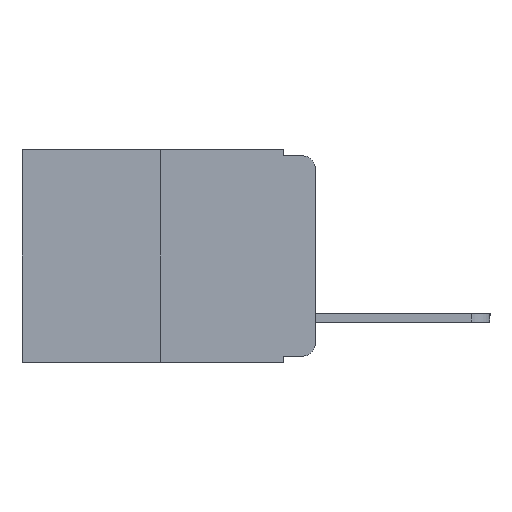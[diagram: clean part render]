
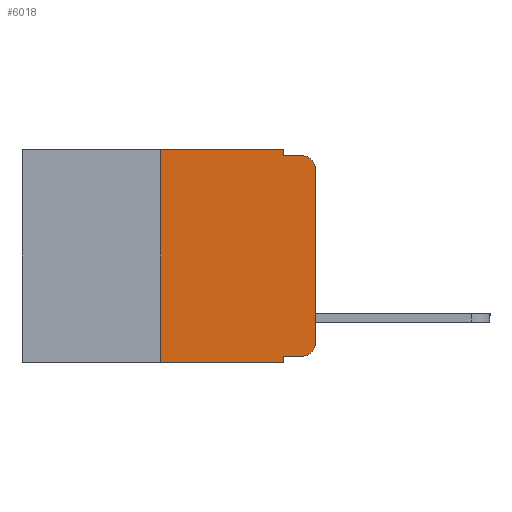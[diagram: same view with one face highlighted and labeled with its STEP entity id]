
A CAD part, left-side view. The second image highlights one B-rep face of the part: STEP entity #6018.
In plain terms, the highlighted planar face has unit normal (-1, 0, 0).
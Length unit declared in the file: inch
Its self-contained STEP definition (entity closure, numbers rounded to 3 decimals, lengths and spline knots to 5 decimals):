
#247 = ORIENTED_EDGE ( 'NONE', *, *, #2678, .F. ) ;
#1972 = LINE ( 'NONE', #10552, #6035 ) ;
#2159 = EDGE_CURVE ( 'NONE', #5291, #13339, #17502, .T. ) ;
#2194 = EDGE_CURVE ( 'NONE', #17381, #5291, #2397, .T. ) ;
#2248 = EDGE_CURVE ( 'NONE', #17381, #13971, #9463, .T. ) ;
#2251 = EDGE_CURVE ( 'NONE', #16331, #6936, #5958, .T. ) ;
#2273 = EDGE_CURVE ( 'NONE', #5850, #3228, #5027, .T. ) ;
#2397 = LINE ( 'NONE', #7109, #9899 ) ;
#2626 = CARTESIAN_POINT ( 'NONE',  ( 0., 0.473, 0. ) ) ;
#2678 = EDGE_CURVE ( 'NONE', #3228, #6550, #5731, .T. ) ;
#2682 = EDGE_CURVE ( 'NONE', #3703, #6550, #12694, .T. ) ;
#2685 = EDGE_CURVE ( 'NONE', #13339, #3703, #5261, .T. ) ;
#3228 = VERTEX_POINT ( 'NONE', #13701 ) ;
#3464 = CARTESIAN_POINT ( 'NONE',  ( 0., 0.02, -0.333 ) ) ;
#3703 = VERTEX_POINT ( 'NONE', #9690 ) ;
#3707 = CARTESIAN_POINT ( 'NONE',  ( 0., 0.051, -0.343 ) ) ;
#3826 = DIRECTION ( 'NONE',  ( 0., 0., -1. ) ) ;
#4146 = DIRECTION ( 'NONE',  ( 0., -1., 0. ) ) ;
#4925 = DIRECTION ( 'NONE',  ( 0., 0., 1. ) ) ;
#5027 = LINE ( 'NONE', #6046, #15476 ) ;
#5111 = CARTESIAN_POINT ( 'NONE',  ( 0., 0.25, 0. ) ) ;
#5170 = DIRECTION ( 'NONE',  ( 0., 0., -1. ) ) ;
#5261 = LINE ( 'NONE', #17087, #15670 ) ;
#5291 = VERTEX_POINT ( 'NONE', #3464 ) ;
#5731 = LINE ( 'NONE', #8336, #9234 ) ;
#5735 = CARTESIAN_POINT ( 'NONE',  ( 0., 0.25, 0. ) ) ;
#5850 = VERTEX_POINT ( 'NONE', #5943 ) ;
#5943 = CARTESIAN_POINT ( 'NONE',  ( 0., 0.051, 0. ) ) ;
#5949 = CARTESIAN_POINT ( 'NONE',  ( 0., 0.25, -0.343 ) ) ;
#5958 = LINE ( 'NONE', #5111, #9007 ) ;
#6018 = ADVANCED_FACE ( 'NONE', ( #11498 ), #15087, .F. ) ;
#6035 = VECTOR ( 'NONE', #9173, 39.37008 ) ;
#6046 = CARTESIAN_POINT ( 'NONE',  ( 0., 0.051, 0. ) ) ;
#6058 = CARTESIAN_POINT ( 'NONE',  ( 0., 0.051, 0. ) ) ;
#6550 = VERTEX_POINT ( 'NONE', #13350 ) ;
#6936 = VERTEX_POINT ( 'NONE', #5735 ) ;
#7101 = EDGE_CURVE ( 'NONE', #16331, #13971, #1972, .T. ) ;
#7109 = CARTESIAN_POINT ( 'NONE',  ( 0., 0.051, -0.333 ) ) ;
#7157 = VECTOR ( 'NONE', #13172, 39.37008 ) ;
#7389 = DIRECTION ( 'NONE',  ( 0., -1., 0. ) ) ;
#7745 = EDGE_LOOP ( 'NONE', ( #14069, #11121, #247, #14455, #15666, #8746, #9229, #9391, #16634, #12688 ) ) ;
#7762 = DIRECTION ( 'NONE',  ( 0., 0., -1. ) ) ;
#7802 = DIRECTION ( 'NONE',  ( -1., 0., 0. ) ) ;
#7881 = CARTESIAN_POINT ( 'NONE',  ( 0., 0.02, -0.313 ) ) ;
#8336 = CARTESIAN_POINT ( 'NONE',  ( 0., 0.051, -0.01 ) ) ;
#8705 = AXIS2_PLACEMENT_3D ( 'NONE', #2626, #15027, #15004 ) ;
#8746 = ORIENTED_EDGE ( 'NONE', *, *, #2251, .F. ) ;
#9007 = VECTOR ( 'NONE', #4925, 39.37008 ) ;
#9173 = DIRECTION ( 'NONE',  ( 0., -1., 0. ) ) ;
#9229 = ORIENTED_EDGE ( 'NONE', *, *, #7101, .T. ) ;
#9234 = VECTOR ( 'NONE', #4146, 39.37008 ) ;
#9391 = ORIENTED_EDGE ( 'NONE', *, *, #2248, .F. ) ;
#9463 = LINE ( 'NONE', #6058, #15874 ) ;
#9690 = CARTESIAN_POINT ( 'NONE',  ( 0., 0., -0.03 ) ) ;
#9899 = VECTOR ( 'NONE', #7389, 39.37008 ) ;
#10214 = AXIS2_PLACEMENT_3D ( 'NONE', #7881, #7802, #7762 ) ;
#10552 = CARTESIAN_POINT ( 'NONE',  ( 0., 0.473, -0.343 ) ) ;
#11121 = ORIENTED_EDGE ( 'NONE', *, *, #2682, .T. ) ;
#11498 = FACE_OUTER_BOUND ( 'NONE', #7745, .T. ) ;
#11876 = CARTESIAN_POINT ( 'NONE',  ( 0., 0.473, 0. ) ) ;
#12107 = DIRECTION ( 'NONE',  ( 0., 0., 1. ) ) ;
#12430 = EDGE_CURVE ( 'NONE', #6936, #5850, #14701, .T. ) ;
#12511 = CARTESIAN_POINT ( 'NONE',  ( 0., 0.051, -0.333 ) ) ;
#12688 = ORIENTED_EDGE ( 'NONE', *, *, #2159, .T. ) ;
#12694 = CIRCLE ( 'NONE', #15323, 0.02 ) ;
#12994 = CARTESIAN_POINT ( 'NONE',  ( 0., 0., -0.313 ) ) ;
#13172 = DIRECTION ( 'NONE',  ( 0., -1., 0. ) ) ;
#13339 = VERTEX_POINT ( 'NONE', #12994 ) ;
#13350 = CARTESIAN_POINT ( 'NONE',  ( 0., 0.02, -0.01 ) ) ;
#13701 = CARTESIAN_POINT ( 'NONE',  ( 0., 0.051, -0.01 ) ) ;
#13971 = VERTEX_POINT ( 'NONE', #3707 ) ;
#14069 = ORIENTED_EDGE ( 'NONE', *, *, #2685, .T. ) ;
#14455 = ORIENTED_EDGE ( 'NONE', *, *, #2273, .F. ) ;
#14701 = LINE ( 'NONE', #11876, #7157 ) ;
#15004 = DIRECTION ( 'NONE',  ( 0., 0., -1. ) ) ;
#15027 = DIRECTION ( 'NONE',  ( 1., 0., 0. ) ) ;
#15087 = PLANE ( 'NONE',  #8705 ) ;
#15323 = AXIS2_PLACEMENT_3D ( 'NONE', #16912, #17704, #17763 ) ;
#15476 = VECTOR ( 'NONE', #3826, 39.37008 ) ;
#15666 = ORIENTED_EDGE ( 'NONE', *, *, #12430, .F. ) ;
#15670 = VECTOR ( 'NONE', #12107, 39.37008 ) ;
#15874 = VECTOR ( 'NONE', #5170, 39.37008 ) ;
#16331 = VERTEX_POINT ( 'NONE', #5949 ) ;
#16634 = ORIENTED_EDGE ( 'NONE', *, *, #2194, .T. ) ;
#16912 = CARTESIAN_POINT ( 'NONE',  ( 0., 0.02, -0.03 ) ) ;
#17087 = CARTESIAN_POINT ( 'NONE',  ( 0., 0., 0. ) ) ;
#17381 = VERTEX_POINT ( 'NONE', #12511 ) ;
#17502 = CIRCLE ( 'NONE', #10214, 0.02 ) ;
#17704 = DIRECTION ( 'NONE',  ( -1., 0., 0. ) ) ;
#17763 = DIRECTION ( 'NONE',  ( 0., 0., -1. ) ) ;
